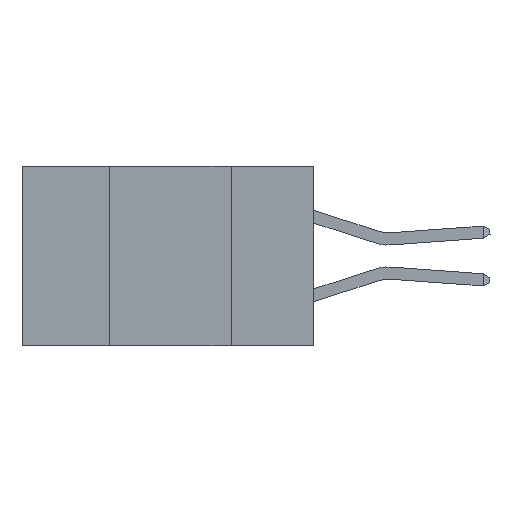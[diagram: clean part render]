
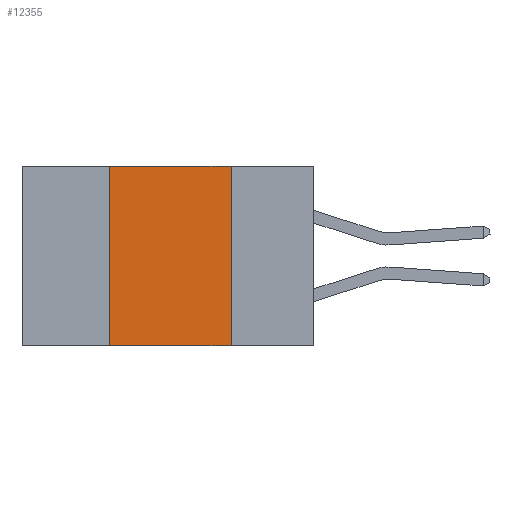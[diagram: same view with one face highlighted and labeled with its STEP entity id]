
A CAD part, left-side view. The second image highlights one B-rep face of the part: STEP entity #12355.
In plain terms, the highlighted planar face has unit normal (-1, 0, 0).
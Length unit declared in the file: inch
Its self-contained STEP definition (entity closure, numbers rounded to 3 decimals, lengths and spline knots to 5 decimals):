
#450 = EDGE_CURVE ( 'NONE', #4094, #14712, #20808, .T. ) ;
#1643 = ORIENTED_EDGE ( 'NONE', *, *, #450, .F. ) ;
#2820 = AXIS2_PLACEMENT_3D ( 'NONE', #12456, #19045, #27863 ) ;
#3358 = EDGE_CURVE ( 'NONE', #17114, #4094, #6764, .T. ) ;
#4094 = VERTEX_POINT ( 'NONE', #21065 ) ;
#4111 = FACE_OUTER_BOUND ( 'NONE', #25034, .T. ) ;
#4165 = CARTESIAN_POINT ( 'NONE',  ( 0., 0.42, 0. ) ) ;
#5306 = VERTEX_POINT ( 'NONE', #23650 ) ;
#5739 = VECTOR ( 'NONE', #19007, 39.37008 ) ;
#5771 = EDGE_CURVE ( 'NONE', #17114, #5306, #10944, .T. ) ;
#6029 = ORIENTED_EDGE ( 'NONE', *, *, #3358, .F. ) ;
#6764 = LINE ( 'NONE', #4165, #12852 ) ;
#10857 = PLANE ( 'NONE',  #2820 ) ;
#10944 = LINE ( 'NONE', #15821, #15218 ) ;
#12355 = ADVANCED_FACE ( 'NONE', ( #4111 ), #10857, .F. ) ;
#12456 = CARTESIAN_POINT ( 'NONE',  ( 0., 0.6, 0. ) ) ;
#12696 = ORIENTED_EDGE ( 'NONE', *, *, #5771, .T. ) ;
#12852 = VECTOR ( 'NONE', #17356, 39.37008 ) ;
#13185 = CARTESIAN_POINT ( 'NONE',  ( 0., 0.42, -0.37 ) ) ;
#14712 = VERTEX_POINT ( 'NONE', #16840 ) ;
#15218 = VECTOR ( 'NONE', #19704, 39.37008 ) ;
#15821 = CARTESIAN_POINT ( 'NONE',  ( 0., 0.6, -0.37 ) ) ;
#16840 = CARTESIAN_POINT ( 'NONE',  ( 0., 0.17, 0. ) ) ;
#17114 = VERTEX_POINT ( 'NONE', #13185 ) ;
#17120 = LINE ( 'NONE', #25513, #5739 ) ;
#17356 = DIRECTION ( 'NONE',  ( 0., 0., 1. ) ) ;
#18739 = EDGE_CURVE ( 'NONE', #14712, #5306, #17120, .T. ) ;
#18778 = DIRECTION ( 'NONE',  ( 0., -1., 0. ) ) ;
#19007 = DIRECTION ( 'NONE',  ( 0., 0., -1. ) ) ;
#19045 = DIRECTION ( 'NONE',  ( 1., 0., 0. ) ) ;
#19704 = DIRECTION ( 'NONE',  ( 0., -1., 0. ) ) ;
#20808 = LINE ( 'NONE', #23122, #28314 ) ;
#21065 = CARTESIAN_POINT ( 'NONE',  ( 0., 0.42, 0. ) ) ;
#23109 = ORIENTED_EDGE ( 'NONE', *, *, #18739, .F. ) ;
#23122 = CARTESIAN_POINT ( 'NONE',  ( 0., 0.6, 0. ) ) ;
#23650 = CARTESIAN_POINT ( 'NONE',  ( 0., 0.17, -0.37 ) ) ;
#25034 = EDGE_LOOP ( 'NONE', ( #23109, #1643, #6029, #12696 ) ) ;
#25513 = CARTESIAN_POINT ( 'NONE',  ( 0., 0.17, 0. ) ) ;
#27863 = DIRECTION ( 'NONE',  ( 0., 0., -1. ) ) ;
#28314 = VECTOR ( 'NONE', #18778, 39.37008 ) ;
